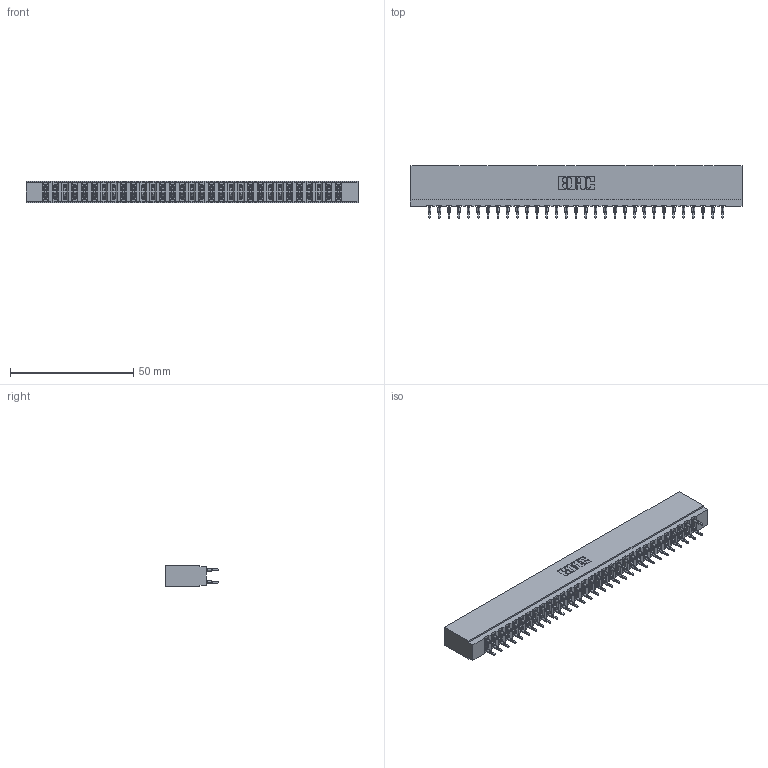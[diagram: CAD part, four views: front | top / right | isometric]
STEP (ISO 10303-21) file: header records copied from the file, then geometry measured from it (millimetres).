
FILE_DESCRIPTION (( 'STEP AP203' ), '1' );
FILE_NAME ('737-062-560-201.STEP', '2020-09-11T06:08:01', ( '' ), ( '' ), 'SwSTEP 2.0', 'SolidWorks 2020', '' );
FILE_SCHEMA (( 'CONFIG_CONTROL_DESIGN' ));
Length unit declared in the file: inch
Products named in the file (3): 737 Part_Insulator Option - 01; 737-062-560-201; 745-292-001_560
Assembly tree (63 placements, depth 2):
  737-062-560-201
    737 Part_Insulator Option - 01
    745-292-001_560  x62
Bounding box: 134.67 x 21.22 x 8.89 mm (x, y, z)
Volume: 13609.8 mm3; surface area: 20637.9 mm2
Topology: 63 solids, 63 shells, 6232 faces, 17057 edges, 10834 vertices
Faces by surface type: plane 3247, cylinder 1373, bspline 1240, torus 372
Entity records: 55010 total; most frequent: CARTESIAN_POINT 10057, ORIENTED_EDGE 9470, DIRECTION 8279, EDGE_CURVE 4735, VECTOR 4359, LINE 4359, VERTEX_POINT 3026, AXIS2_PLACEMENT_3D 1960
